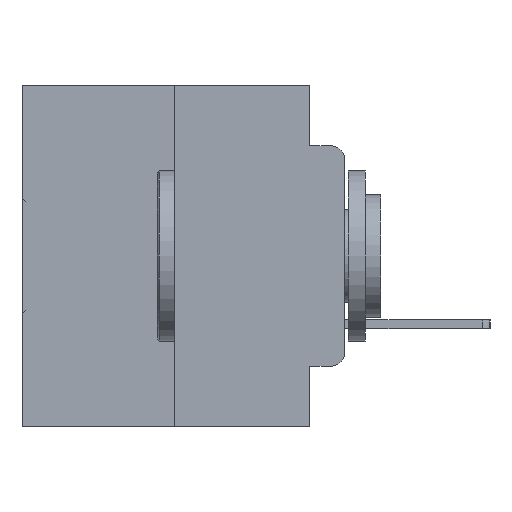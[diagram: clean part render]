
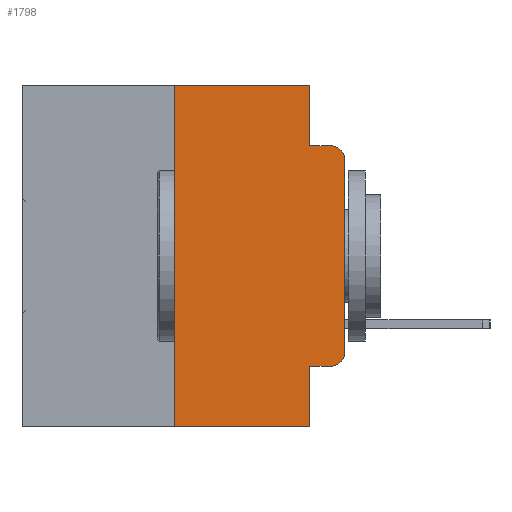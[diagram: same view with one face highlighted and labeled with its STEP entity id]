
A CAD part, left-side view. The second image highlights one B-rep face of the part: STEP entity #1798.
In plain terms, the highlighted planar face has unit normal (-1, 0, 0).
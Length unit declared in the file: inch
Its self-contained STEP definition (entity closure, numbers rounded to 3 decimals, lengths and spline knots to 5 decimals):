
#323 = CARTESIAN_POINT ( 'NONE',  ( 0., 0., -0.1085 ) ) ;
#381 = EDGE_CURVE ( 'NONE', #7010, #10578, #7065, .T. ) ;
#1499 = LINE ( 'NONE', #10938, #26327 ) ;
#1671 = AXIS2_PLACEMENT_3D ( 'NONE', #22121, #19991, #5697 ) ;
#1798 = ADVANCED_FACE ( 'NONE', ( #29057 ), #2999, .F. ) ;
#1817 = ORIENTED_EDGE ( 'NONE', *, *, #12769, .F. ) ;
#1951 = EDGE_CURVE ( 'NONE', #27487, #18687, #29417, .T. ) ;
#2242 = ORIENTED_EDGE ( 'NONE', *, *, #2668, .F. ) ;
#2668 = EDGE_CURVE ( 'NONE', #28716, #20137, #8068, .T. ) ;
#2999 = PLANE ( 'NONE',  #1671 ) ;
#3570 = VECTOR ( 'NONE', #19261, 39.37008 ) ;
#4166 = CARTESIAN_POINT ( 'NONE',  ( 0., 0.051, -0.5 ) ) ;
#4644 = DIRECTION ( 'NONE',  ( -1., 0., 0. ) ) ;
#4872 = EDGE_CURVE ( 'NONE', #20459, #27487, #10209, .T. ) ;
#4879 = CARTESIAN_POINT ( 'NONE',  ( 0., 0.051, 0. ) ) ;
#5126 = EDGE_CURVE ( 'NONE', #8521, #28716, #1499, .T. ) ;
#5170 = DIRECTION ( 'NONE',  ( 0., -1., 0. ) ) ;
#5697 = DIRECTION ( 'NONE',  ( 0., 0., -1. ) ) ;
#6004 = DIRECTION ( 'NONE',  ( 0., 0., 1. ) ) ;
#6158 = EDGE_CURVE ( 'NONE', #6758, #18687, #6595, .T. ) ;
#6595 = LINE ( 'NONE', #14833, #23982 ) ;
#6653 = ORIENTED_EDGE ( 'NONE', *, *, #24396, .T. ) ;
#6758 = VERTEX_POINT ( 'NONE', #27240 ) ;
#7010 = VERTEX_POINT ( 'NONE', #14167 ) ;
#7065 = LINE ( 'NONE', #19858, #25145 ) ;
#7446 = DIRECTION ( 'NONE',  ( 0., 0., -1. ) ) ;
#7868 = DIRECTION ( 'NONE',  ( 0., 0., -1. ) ) ;
#8068 = LINE ( 'NONE', #12163, #14415 ) ;
#8190 = CARTESIAN_POINT ( 'NONE',  ( 0., 0.02, -0.0885 ) ) ;
#8521 = VERTEX_POINT ( 'NONE', #9951 ) ;
#8869 = CARTESIAN_POINT ( 'NONE',  ( 0., 0.02, -0.1085 ) ) ;
#9750 = VECTOR ( 'NONE', #9872, 39.37008 ) ;
#9872 = DIRECTION ( 'NONE',  ( 0., -1., 0. ) ) ;
#9951 = CARTESIAN_POINT ( 'NONE',  ( 0., 0.25, -0.5 ) ) ;
#10209 = LINE ( 'NONE', #28539, #3570 ) ;
#10578 = VERTEX_POINT ( 'NONE', #22922 ) ;
#10938 = CARTESIAN_POINT ( 'NONE',  ( 0., 0.25, 0. ) ) ;
#11221 = ORIENTED_EDGE ( 'NONE', *, *, #1951, .T. ) ;
#11261 = DIRECTION ( 'NONE',  ( 0., 0., -1. ) ) ;
#11506 = CARTESIAN_POINT ( 'NONE',  ( 0., 0.051, 0. ) ) ;
#12163 = CARTESIAN_POINT ( 'NONE',  ( 0., 0.473, 0. ) ) ;
#12709 = ORIENTED_EDGE ( 'NONE', *, *, #31014, .T. ) ;
#12769 = EDGE_CURVE ( 'NONE', #20137, #6758, #19764, .T. ) ;
#12872 = LINE ( 'NONE', #4879, #19060 ) ;
#13128 = VERTEX_POINT ( 'NONE', #4166 ) ;
#14167 = CARTESIAN_POINT ( 'NONE',  ( 0., 0.051, -0.4115 ) ) ;
#14294 = VECTOR ( 'NONE', #7868, 39.37008 ) ;
#14415 = VECTOR ( 'NONE', #26170, 39.37008 ) ;
#14833 = CARTESIAN_POINT ( 'NONE',  ( 0., 0.051, -0.0885 ) ) ;
#16384 = ORIENTED_EDGE ( 'NONE', *, *, #29079, .F. ) ;
#16543 = AXIS2_PLACEMENT_3D ( 'NONE', #8869, #25277, #11261 ) ;
#17449 = ORIENTED_EDGE ( 'NONE', *, *, #5126, .F. ) ;
#18687 = VERTEX_POINT ( 'NONE', #8190 ) ;
#19003 = CARTESIAN_POINT ( 'NONE',  ( 0., 0.02, -0.3915 ) ) ;
#19060 = VECTOR ( 'NONE', #7446, 39.37008 ) ;
#19261 = DIRECTION ( 'NONE',  ( 0., 0., 1. ) ) ;
#19764 = LINE ( 'NONE', #24333, #14294 ) ;
#19816 = DIRECTION ( 'NONE',  ( 0., -1., 0. ) ) ;
#19858 = CARTESIAN_POINT ( 'NONE',  ( 0., 0.051, -0.4115 ) ) ;
#19991 = DIRECTION ( 'NONE',  ( 1., 0., 0. ) ) ;
#20137 = VERTEX_POINT ( 'NONE', #11506 ) ;
#20459 = VERTEX_POINT ( 'NONE', #22109 ) ;
#20893 = EDGE_LOOP ( 'NONE', ( #21464, #11221, #29880, #1817, #2242, #17449, #12709, #16384, #23309, #6653 ) ) ;
#21369 = DIRECTION ( 'NONE',  ( 0., 0., -1. ) ) ;
#21464 = ORIENTED_EDGE ( 'NONE', *, *, #4872, .T. ) ;
#22109 = CARTESIAN_POINT ( 'NONE',  ( 0., 0., -0.3915 ) ) ;
#22121 = CARTESIAN_POINT ( 'NONE',  ( 0., 0.473, 0. ) ) ;
#22922 = CARTESIAN_POINT ( 'NONE',  ( 0., 0.02, -0.4115 ) ) ;
#23309 = ORIENTED_EDGE ( 'NONE', *, *, #381, .T. ) ;
#23982 = VECTOR ( 'NONE', #5170, 39.37008 ) ;
#24333 = CARTESIAN_POINT ( 'NONE',  ( 0., 0.051, 0. ) ) ;
#24396 = EDGE_CURVE ( 'NONE', #10578, #20459, #27104, .T. ) ;
#25145 = VECTOR ( 'NONE', #19816, 39.37008 ) ;
#25277 = DIRECTION ( 'NONE',  ( -1., 0., 0. ) ) ;
#26170 = DIRECTION ( 'NONE',  ( 0., -1., 0. ) ) ;
#26282 = CARTESIAN_POINT ( 'NONE',  ( 0., 0.473, -0.5 ) ) ;
#26327 = VECTOR ( 'NONE', #6004, 39.37008 ) ;
#27014 = AXIS2_PLACEMENT_3D ( 'NONE', #19003, #4644, #21369 ) ;
#27104 = CIRCLE ( 'NONE', #27014, 0.02 ) ;
#27234 = CARTESIAN_POINT ( 'NONE',  ( 0., 0.25, 0. ) ) ;
#27240 = CARTESIAN_POINT ( 'NONE',  ( 0., 0.051, -0.0885 ) ) ;
#27487 = VERTEX_POINT ( 'NONE', #323 ) ;
#28432 = LINE ( 'NONE', #26282, #9750 ) ;
#28539 = CARTESIAN_POINT ( 'NONE',  ( 0., 0., 0. ) ) ;
#28716 = VERTEX_POINT ( 'NONE', #27234 ) ;
#29057 = FACE_OUTER_BOUND ( 'NONE', #20893, .T. ) ;
#29079 = EDGE_CURVE ( 'NONE', #7010, #13128, #12872, .T. ) ;
#29417 = CIRCLE ( 'NONE', #16543, 0.02 ) ;
#29880 = ORIENTED_EDGE ( 'NONE', *, *, #6158, .F. ) ;
#31014 = EDGE_CURVE ( 'NONE', #8521, #13128, #28432, .T. ) ;
